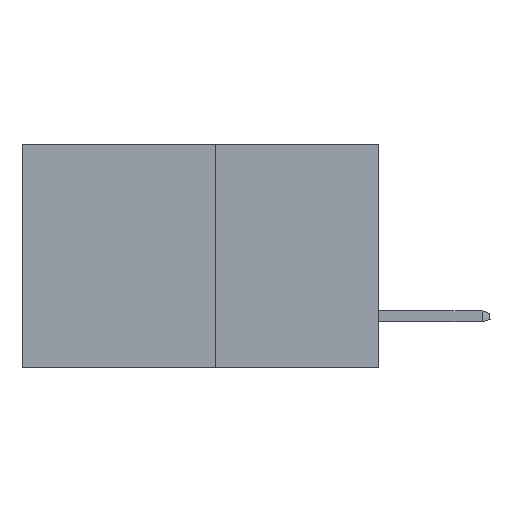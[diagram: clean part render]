
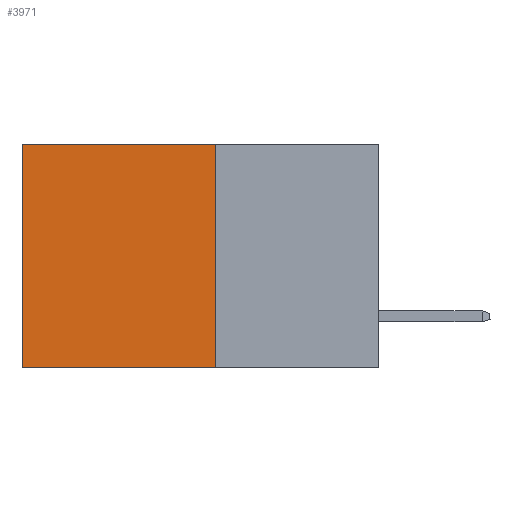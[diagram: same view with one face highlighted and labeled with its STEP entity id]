
A CAD part, left-side view. The second image highlights one B-rep face of the part: STEP entity #3971.
In plain terms, the highlighted planar face has unit normal (-1, 0, 0).
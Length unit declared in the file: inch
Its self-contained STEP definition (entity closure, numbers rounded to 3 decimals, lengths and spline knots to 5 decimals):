
#155 = DIRECTION ( 'NONE',  ( 0., 0., -1. ) ) ;
#361 = EDGE_CURVE ( 'NONE', #6433, #5801, #8995, .T. ) ;
#369 = DIRECTION ( 'NONE',  ( 0., 1., 0. ) ) ;
#442 = ORIENTED_EDGE ( 'NONE', *, *, #361, .T. ) ;
#504 = CARTESIAN_POINT ( 'NONE',  ( 0.277, 0.27, -0.37 ) ) ;
#1642 = EDGE_LOOP ( 'NONE', ( #4491, #7182, #9810, #442 ) ) ;
#2027 = VECTOR ( 'NONE', #7890, 39.37008 ) ;
#2764 = DIRECTION ( 'NONE',  ( 0., 1., 0. ) ) ;
#2862 = DIRECTION ( 'NONE',  ( 0., 0., -1. ) ) ;
#2950 = DIRECTION ( 'NONE',  ( 1., 0., 0. ) ) ;
#3008 = VERTEX_POINT ( 'NONE', #7838 ) ;
#3255 = VECTOR ( 'NONE', #369, 39.37008 ) ;
#3292 = PLANE ( 'NONE',  #3338 ) ;
#3338 = AXIS2_PLACEMENT_3D ( 'NONE', #5864, #2950, #2862 ) ;
#3533 = LINE ( 'NONE', #504, #3255 ) ;
#3717 = CARTESIAN_POINT ( 'NONE',  ( 0.277, 0.27, 0. ) ) ;
#3971 = ADVANCED_FACE ( 'NONE', ( #9084 ), #3292, .F. ) ;
#4235 = LINE ( 'NONE', #7899, #2027 ) ;
#4491 = ORIENTED_EDGE ( 'NONE', *, *, #8008, .T. ) ;
#5525 = EDGE_CURVE ( 'NONE', #6786, #3008, #3533, .T. ) ;
#5743 = EDGE_CURVE ( 'NONE', #6433, #6786, #10558, .T. ) ;
#5801 = VERTEX_POINT ( 'NONE', #7670 ) ;
#5864 = CARTESIAN_POINT ( 'NONE',  ( 0.277, 0.27, -0.37 ) ) ;
#6429 = CARTESIAN_POINT ( 'NONE',  ( 0.277, 0.27, 0. ) ) ;
#6433 = VERTEX_POINT ( 'NONE', #3717 ) ;
#6786 = VERTEX_POINT ( 'NONE', #7297 ) ;
#7182 = ORIENTED_EDGE ( 'NONE', *, *, #5525, .F. ) ;
#7297 = CARTESIAN_POINT ( 'NONE',  ( 0.277, 0.27, -0.37 ) ) ;
#7670 = CARTESIAN_POINT ( 'NONE',  ( 0.277, 0.59, 0. ) ) ;
#7838 = CARTESIAN_POINT ( 'NONE',  ( 0.277, 0.59, -0.37 ) ) ;
#7890 = DIRECTION ( 'NONE',  ( 0., 0., -1. ) ) ;
#7899 = CARTESIAN_POINT ( 'NONE',  ( 0.277, 0.59, -0.37 ) ) ;
#8008 = EDGE_CURVE ( 'NONE', #5801, #3008, #4235, .T. ) ;
#8715 = VECTOR ( 'NONE', #2764, 39.37008 ) ;
#8995 = LINE ( 'NONE', #6429, #8715 ) ;
#9084 = FACE_OUTER_BOUND ( 'NONE', #1642, .T. ) ;
#9810 = ORIENTED_EDGE ( 'NONE', *, *, #5743, .F. ) ;
#10089 = CARTESIAN_POINT ( 'NONE',  ( 0.277, 0.27, -0.37 ) ) ;
#10558 = LINE ( 'NONE', #10089, #10832 ) ;
#10832 = VECTOR ( 'NONE', #155, 39.37008 ) ;
